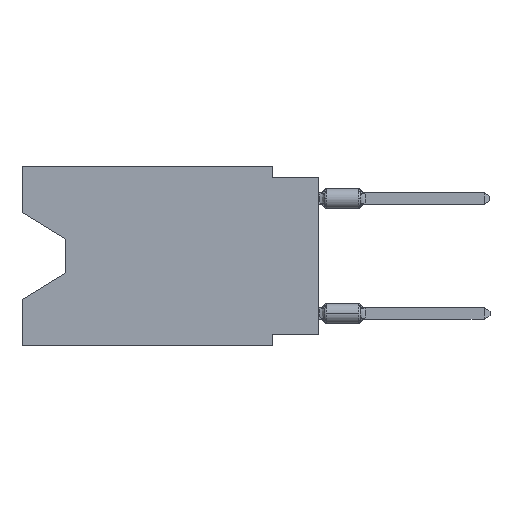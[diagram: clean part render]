
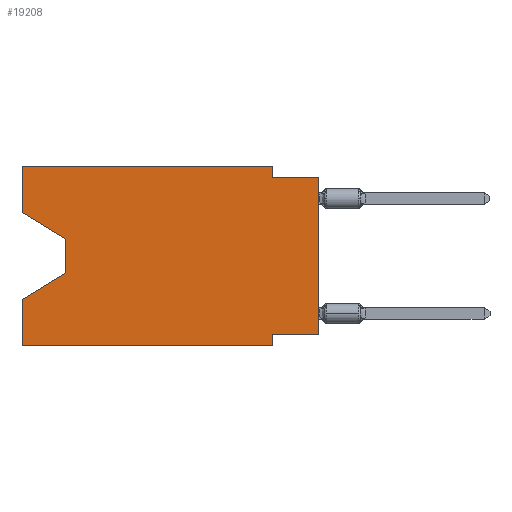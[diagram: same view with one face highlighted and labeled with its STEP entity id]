
A CAD part, left-side view. The second image highlights one B-rep face of the part: STEP entity #19208.
In plain terms, the highlighted planar face has unit normal (-1, 0, 0).
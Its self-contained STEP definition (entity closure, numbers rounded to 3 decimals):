
#58 = VERTEX_POINT ( 'NONE', #7468 ) ;
#522 = VERTEX_POINT ( 'NONE', #6050 ) ;
#739 = VERTEX_POINT ( 'NONE', #12355 ) ;
#1050 = EDGE_CURVE ( 'NONE', #12356, #21252, #1146, .T. ) ;
#1137 = EDGE_CURVE ( 'NONE', #58, #16450, #10812, .T. ) ;
#1146 = LINE ( 'NONE', #13367, #5957 ) ;
#1731 = VERTEX_POINT ( 'NONE', #19915 ) ;
#1867 = ORIENTED_EDGE ( 'NONE', *, *, #4862, .F. ) ;
#2056 = VECTOR ( 'NONE', #2080, 1000. ) ;
#2080 = DIRECTION ( 'NONE',  ( 0., -0.855, -0.519 ) ) ;
#2243 = CARTESIAN_POINT ( 'NONE',  ( 0., 0., -9.271 ) ) ;
#2244 = VERTEX_POINT ( 'NONE', #12239 ) ;
#2460 = DIRECTION ( 'NONE',  ( 0., 0., 1. ) ) ;
#2756 = LINE ( 'NONE', #9991, #4545 ) ;
#2980 = DIRECTION ( 'NONE',  ( 0., -1., 0. ) ) ;
#3308 = VERTEX_POINT ( 'NONE', #4504 ) ;
#3896 = EDGE_CURVE ( 'NONE', #16450, #12356, #19251, .T. ) ;
#3998 = DIRECTION ( 'NONE',  ( 0., 0., -1. ) ) ;
#4334 = DIRECTION ( 'NONE',  ( 0., 0., 1. ) ) ;
#4504 = CARTESIAN_POINT ( 'NONE',  ( 0., 13.97, -4.013 ) ) ;
#4512 = ORIENTED_EDGE ( 'NONE', *, *, #8974, .T. ) ;
#4545 = VECTOR ( 'NONE', #2980, 1000. ) ;
#4639 = VERTEX_POINT ( 'NONE', #22512 ) ;
#4850 = VECTOR ( 'NONE', #10701, 1000. ) ;
#4862 = EDGE_CURVE ( 'NONE', #21343, #58, #21377, .T. ) ;
#5009 = ORIENTED_EDGE ( 'NONE', *, *, #21918, .F. ) ;
#5500 = ORIENTED_EDGE ( 'NONE', *, *, #1050, .F. ) ;
#5557 = CARTESIAN_POINT ( 'NONE',  ( 0., 0., 0. ) ) ;
#5671 = CARTESIAN_POINT ( 'NONE',  ( 0., 13.97, -5.893 ) ) ;
#5957 = VECTOR ( 'NONE', #20869, 1000. ) ;
#6050 = CARTESIAN_POINT ( 'NONE',  ( 0., 16.383, -9.906 ) ) ;
#6124 = VECTOR ( 'NONE', #3998, 1000. ) ;
#6511 = LINE ( 'NONE', #9862, #19775 ) ;
#6517 = ORIENTED_EDGE ( 'NONE', *, *, #8047, .T. ) ;
#6585 = CARTESIAN_POINT ( 'NONE',  ( 0., 2.54, -9.906 ) ) ;
#7223 = VECTOR ( 'NONE', #16215, 1000. ) ;
#7272 = PLANE ( 'NONE',  #9014 ) ;
#7468 = CARTESIAN_POINT ( 'NONE',  ( 0., 16.383, 0. ) ) ;
#7932 = VECTOR ( 'NONE', #10990, 1000. ) ;
#8047 = EDGE_CURVE ( 'NONE', #739, #21252, #21494, .T. ) ;
#8071 = EDGE_CURVE ( 'NONE', #739, #20470, #9253, .T. ) ;
#8194 = DIRECTION ( 'NONE',  ( 0., 0., -1. ) ) ;
#8473 = ORIENTED_EDGE ( 'NONE', *, *, #21834, .T. ) ;
#8711 = CARTESIAN_POINT ( 'NONE',  ( 0., 16.383, -2.546 ) ) ;
#8974 = EDGE_CURVE ( 'NONE', #3308, #2244, #16244, .T. ) ;
#9014 = AXIS2_PLACEMENT_3D ( 'NONE', #14067, #21454, #17672 ) ;
#9111 = EDGE_CURVE ( 'NONE', #522, #1731, #6511, .T. ) ;
#9253 = LINE ( 'NONE', #2243, #7932 ) ;
#9862 = CARTESIAN_POINT ( 'NONE',  ( 0., 16.383, 0. ) ) ;
#9991 = CARTESIAN_POINT ( 'NONE',  ( 0., 16.383, -9.906 ) ) ;
#10129 = EDGE_CURVE ( 'NONE', #21343, #3308, #15813, .T. ) ;
#10701 = DIRECTION ( 'NONE',  ( 0., -1., 0. ) ) ;
#10783 = CARTESIAN_POINT ( 'NONE',  ( 0., 2.54, 0. ) ) ;
#10787 = CARTESIAN_POINT ( 'NONE',  ( 0., 13.97, -4.013 ) ) ;
#10812 = LINE ( 'NONE', #19499, #4850 ) ;
#10990 = DIRECTION ( 'NONE',  ( 0., 1., 0. ) ) ;
#11503 = VECTOR ( 'NONE', #2460, 1000. ) ;
#12176 = CARTESIAN_POINT ( 'NONE',  ( 0., 0., -0.635 ) ) ;
#12239 = CARTESIAN_POINT ( 'NONE',  ( 0., 13.97, -5.893 ) ) ;
#12355 = CARTESIAN_POINT ( 'NONE',  ( 0., 0., -9.271 ) ) ;
#12356 = VERTEX_POINT ( 'NONE', #21915 ) ;
#12491 = ORIENTED_EDGE ( 'NONE', *, *, #9111, .F. ) ;
#12635 = ORIENTED_EDGE ( 'NONE', *, *, #1137, .F. ) ;
#13169 = CARTESIAN_POINT ( 'NONE',  ( 0., 16.383, 0. ) ) ;
#13367 = CARTESIAN_POINT ( 'NONE',  ( 0., 0., -0.635 ) ) ;
#13702 = DIRECTION ( 'NONE',  ( 0., 0., -1. ) ) ;
#14067 = CARTESIAN_POINT ( 'NONE',  ( 0., 16.383, 0. ) ) ;
#14363 = ORIENTED_EDGE ( 'NONE', *, *, #17381, .T. ) ;
#15813 = LINE ( 'NONE', #21340, #2056 ) ;
#16109 = VECTOR ( 'NONE', #8194, 1000. ) ;
#16215 = DIRECTION ( 'NONE',  ( 0., 0.855, -0.519 ) ) ;
#16244 = LINE ( 'NONE', #10787, #6124 ) ;
#16450 = VERTEX_POINT ( 'NONE', #10783 ) ;
#16594 = ORIENTED_EDGE ( 'NONE', *, *, #8071, .F. ) ;
#16651 = LINE ( 'NONE', #5671, #7223 ) ;
#17101 = LINE ( 'NONE', #6585, #16109 ) ;
#17381 = EDGE_CURVE ( 'NONE', #522, #4639, #2756, .T. ) ;
#17554 = FACE_OUTER_BOUND ( 'NONE', #19918, .T. ) ;
#17672 = DIRECTION ( 'NONE',  ( 0., 0., -1. ) ) ;
#17674 = CARTESIAN_POINT ( 'NONE',  ( 0., 2.54, -9.271 ) ) ;
#17899 = VECTOR ( 'NONE', #19544, 1000. ) ;
#18782 = ORIENTED_EDGE ( 'NONE', *, *, #3896, .F. ) ;
#19208 = ADVANCED_FACE ( 'NONE', ( #17554 ), #7272, .F. ) ;
#19251 = LINE ( 'NONE', #19373, #21432 ) ;
#19373 = CARTESIAN_POINT ( 'NONE',  ( 0., 2.54, 0. ) ) ;
#19499 = CARTESIAN_POINT ( 'NONE',  ( 0., 16.383, 0. ) ) ;
#19544 = DIRECTION ( 'NONE',  ( 0., 0., 1. ) ) ;
#19775 = VECTOR ( 'NONE', #4334, 1000. ) ;
#19915 = CARTESIAN_POINT ( 'NONE',  ( 0., 16.383, -7.36 ) ) ;
#19918 = EDGE_LOOP ( 'NONE', ( #22648, #4512, #8473, #12491, #14363, #5009, #16594, #6517, #5500, #18782, #12635, #1867 ) ) ;
#20470 = VERTEX_POINT ( 'NONE', #17674 ) ;
#20869 = DIRECTION ( 'NONE',  ( 0., -1., 0. ) ) ;
#21252 = VERTEX_POINT ( 'NONE', #12176 ) ;
#21340 = CARTESIAN_POINT ( 'NONE',  ( 0., 16.383, -2.546 ) ) ;
#21343 = VERTEX_POINT ( 'NONE', #8711 ) ;
#21377 = LINE ( 'NONE', #13169, #11503 ) ;
#21432 = VECTOR ( 'NONE', #13702, 1000. ) ;
#21454 = DIRECTION ( 'NONE',  ( 1., 0., 0. ) ) ;
#21494 = LINE ( 'NONE', #5557, #17899 ) ;
#21834 = EDGE_CURVE ( 'NONE', #2244, #1731, #16651, .T. ) ;
#21915 = CARTESIAN_POINT ( 'NONE',  ( 0., 2.54, -0.635 ) ) ;
#21918 = EDGE_CURVE ( 'NONE', #20470, #4639, #17101, .T. ) ;
#22512 = CARTESIAN_POINT ( 'NONE',  ( 0., 2.54, -9.906 ) ) ;
#22648 = ORIENTED_EDGE ( 'NONE', *, *, #10129, .T. ) ;
